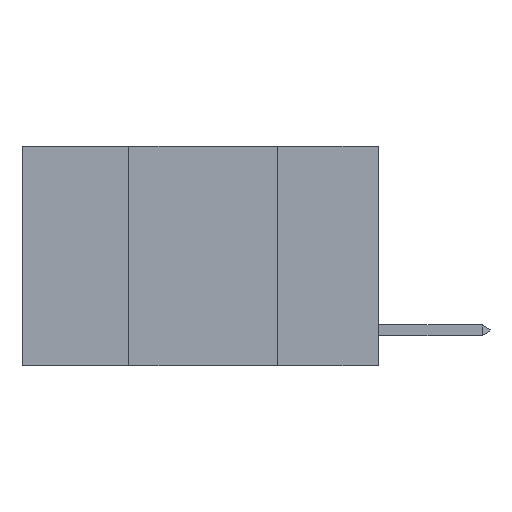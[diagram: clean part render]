
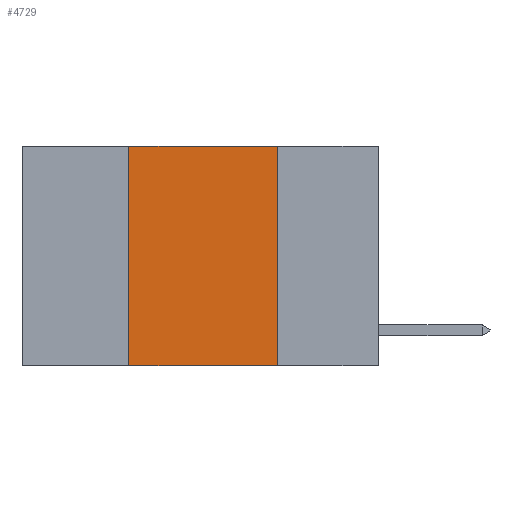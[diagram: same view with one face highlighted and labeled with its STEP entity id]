
A CAD part, left-side view. The second image highlights one B-rep face of the part: STEP entity #4729.
In plain terms, the highlighted planar face has unit normal (-1, 0, 0).
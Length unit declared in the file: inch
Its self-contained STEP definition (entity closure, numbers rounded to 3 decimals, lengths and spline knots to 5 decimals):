
#96 = DIRECTION ( 'NONE',  ( 0., 0., 1. ) ) ;
#512 = LINE ( 'NONE', #4479, #11726 ) ;
#903 = CARTESIAN_POINT ( 'NONE',  ( 0., 0.6, 0. ) ) ;
#1545 = CARTESIAN_POINT ( 'NONE',  ( 0., 0.17, 0. ) ) ;
#1847 = DIRECTION ( 'NONE',  ( 0., 0., -1. ) ) ;
#3026 = PLANE ( 'NONE',  #23886 ) ;
#4458 = EDGE_CURVE ( 'NONE', #12238, #17369, #6719, .T. ) ;
#4479 = CARTESIAN_POINT ( 'NONE',  ( 0., 0.6, -0.37 ) ) ;
#4729 = ADVANCED_FACE ( 'NONE', ( #26901 ), #3026, .F. ) ;
#6269 = ORIENTED_EDGE ( 'NONE', *, *, #11889, .T. ) ;
#6376 = EDGE_LOOP ( 'NONE', ( #11799, #26517, #20696, #6269 ) ) ;
#6719 = LINE ( 'NONE', #25120, #22728 ) ;
#7256 = DIRECTION ( 'NONE',  ( 0., 0., -1. ) ) ;
#9123 = LINE ( 'NONE', #24381, #21628 ) ;
#9242 = EDGE_CURVE ( 'NONE', #17369, #13726, #9123, .T. ) ;
#9609 = CARTESIAN_POINT ( 'NONE',  ( 0., 0.42, 0. ) ) ;
#9725 = VECTOR ( 'NONE', #1847, 39.37008 ) ;
#10083 = CARTESIAN_POINT ( 'NONE',  ( 0., 0.42, -0.37 ) ) ;
#10238 = CARTESIAN_POINT ( 'NONE',  ( 0., 0.17, 0. ) ) ;
#11726 = VECTOR ( 'NONE', #19144, 39.37008 ) ;
#11799 = ORIENTED_EDGE ( 'NONE', *, *, #20096, .F. ) ;
#11889 = EDGE_CURVE ( 'NONE', #12238, #26541, #512, .T. ) ;
#12238 = VERTEX_POINT ( 'NONE', #10083 ) ;
#13726 = VERTEX_POINT ( 'NONE', #1545 ) ;
#17369 = VERTEX_POINT ( 'NONE', #9609 ) ;
#19144 = DIRECTION ( 'NONE',  ( 0., -1., 0. ) ) ;
#19804 = DIRECTION ( 'NONE',  ( 1., 0., 0. ) ) ;
#20096 = EDGE_CURVE ( 'NONE', #13726, #26541, #21483, .T. ) ;
#20696 = ORIENTED_EDGE ( 'NONE', *, *, #4458, .F. ) ;
#21483 = LINE ( 'NONE', #10238, #9725 ) ;
#21628 = VECTOR ( 'NONE', #25368, 39.37008 ) ;
#22728 = VECTOR ( 'NONE', #96, 39.37008 ) ;
#23886 = AXIS2_PLACEMENT_3D ( 'NONE', #903, #19804, #7256 ) ;
#24381 = CARTESIAN_POINT ( 'NONE',  ( 0., 0.6, 0. ) ) ;
#25120 = CARTESIAN_POINT ( 'NONE',  ( 0., 0.42, 0. ) ) ;
#25332 = CARTESIAN_POINT ( 'NONE',  ( 0., 0.17, -0.37 ) ) ;
#25368 = DIRECTION ( 'NONE',  ( 0., -1., 0. ) ) ;
#26517 = ORIENTED_EDGE ( 'NONE', *, *, #9242, .F. ) ;
#26541 = VERTEX_POINT ( 'NONE', #25332 ) ;
#26901 = FACE_OUTER_BOUND ( 'NONE', #6376, .T. ) ;
